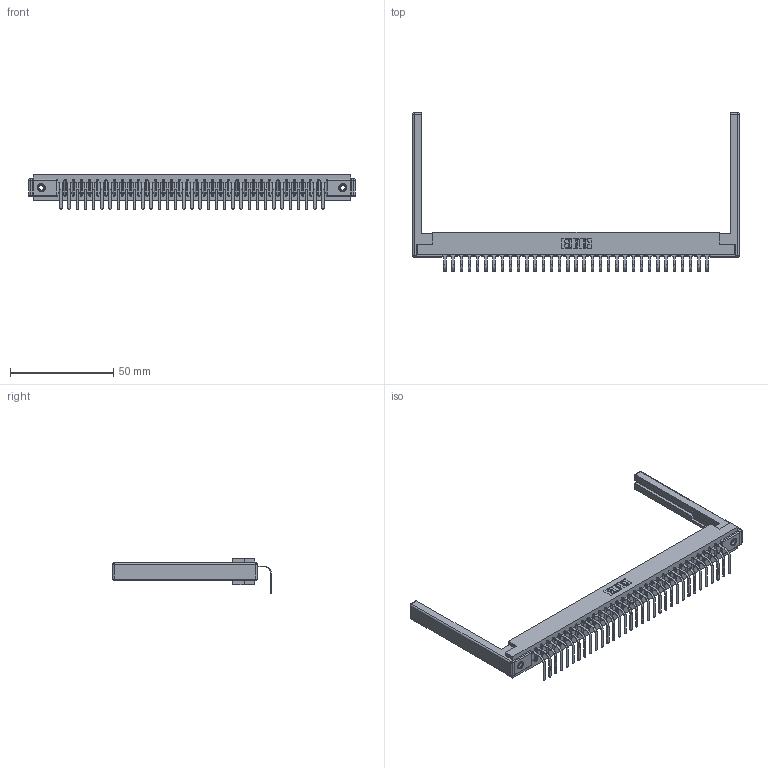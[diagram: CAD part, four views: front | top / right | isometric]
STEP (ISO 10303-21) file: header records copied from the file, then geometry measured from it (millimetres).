
FILE_DESCRIPTION (( 'STEP AP203' ), '1' );
FILE_NAME ('357-033-458-168.STEP', '2022-07-18T20:40:34', ( '' ), ( '' ), 'SwSTEP 2.0', 'SolidWorks 2020', '' );
FILE_SCHEMA (( 'CONFIG_CONTROL_DESIGN' ));
Length unit declared in the file: inch
Products named in the file (5): 357-033-458-168; 307-220-068; 345-250-001_345-250-001-102; 307 Part_.156 Dia Mounting Holes; 307-290-001_558 - 2 (Single)
Assembly tree (38 placements, depth 2):
  357-033-458-168
    307 Part_.156 Dia Mounting Holes
    307-290-001_558 - 2 (Single)  x33
    307-220-068  x2
    345-250-001_345-250-001-102  x2
Bounding box: 158.19 x 76.75 x 16.8 mm (x, y, z)
Volume: 20898.5 mm3; surface area: 22325.5 mm2
Topology: 38 solids, 38 shells, 2286 faces, 6455 edges, 4146 vertices
Faces by surface type: plane 1445, cylinder 749, sphere 76, cone 12, torus 4
Entity records: 32263 total; most frequent: CARTESIAN_POINT 5397, ORIENTED_EDGE 5372, DIRECTION 5272, EDGE_CURVE 2686, VECTOR 2054, LINE 2054, VERTEX_POINT 1734, AXIS2_PLACEMENT_3D 1609
